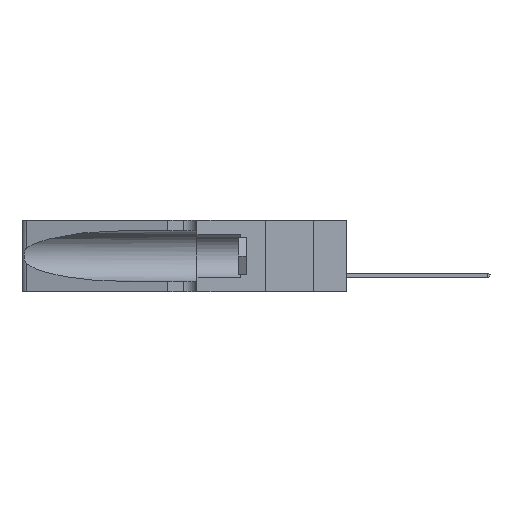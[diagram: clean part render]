
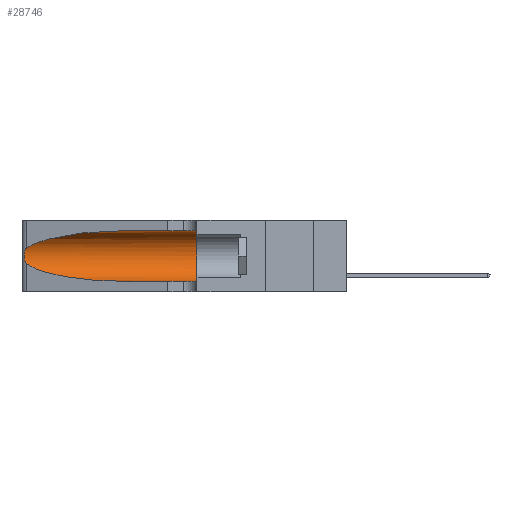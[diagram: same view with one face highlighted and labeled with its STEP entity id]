
A CAD part, left-side view. The second image highlights one B-rep face of the part: STEP entity #28746.
In plain terms, the highlighted cylindrical face has radius 3.308 mm (diameter 6.617 mm), a partial arc.
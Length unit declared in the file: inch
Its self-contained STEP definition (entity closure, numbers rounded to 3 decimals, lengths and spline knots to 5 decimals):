
#509 = DIRECTION ( 'NONE',  ( 0., -1., 0. ) ) ;
#512 = CARTESIAN_POINT ( 'NONE',  ( 0.26017, 1.23833, 0.17102 ) ) ;
#1267 = DIRECTION ( 'NONE',  ( 0., -1., 0. ) ) ;
#1362 = CARTESIAN_POINT ( 'NONE',  ( 0.1305, 1.61858, 0.05475 ) ) ;
#1615 = LINE ( 'NONE', #1362, #5731 ) ;
#3659 = VERTEX_POINT ( 'NONE', #7584 ) ;
#4098 = CARTESIAN_POINT ( 'NONE',  ( 0.1305, 0.35, 0.185 ) ) ;
#4295 = CARTESIAN_POINT ( 'NONE',  ( 0.1305, 0.72297, 0.05475 ) ) ;
#5351 = CARTESIAN_POINT ( 'NONE',  ( 0.25555, 1.22993, 0.14849 ) ) ;
#5681 = CARTESIAN_POINT ( 'NONE',  ( 0.25487, 1.22718, 0.14631 ) ) ;
#5731 = VECTOR ( 'NONE', #1267, 39.37008 ) ;
#5906 = CARTESIAN_POINT ( 'NONE',  ( 0.18966, 0.96281, 0.31525 ) ) ;
#6548 = CARTESIAN_POINT ( 'NONE',  ( 0.25487, 1.22718, 0.22369 ) ) ;
#6645 = CARTESIAN_POINT ( 'NONE',  ( 0.25487, 1.22718, 0.22369 ) ) ;
#6661 =( BOUNDED_CURVE ( )  B_SPLINE_CURVE ( 3, ( #11245, #25977, #30340, #23454 ),
 .UNSPECIFIED., .F., .F. ) 
 B_SPLINE_CURVE_WITH_KNOTS ( ( 4, 4 ),
 ( 3.44316, 4.71239 ),
 .UNSPECIFIED. ) 
 CURVE ( )  GEOMETRIC_REPRESENTATION_ITEM ( )  RATIONAL_B_SPLINE_CURVE ( ( 1., 0.87, 0.87, 1. ) ) 
 REPRESENTATION_ITEM ( '' )  );
#7372 = EDGE_CURVE ( 'NONE', #8222, #18254, #1615, .T. ) ;
#7583 = DIRECTION ( 'NONE',  ( 0., -1., 0. ) ) ;
#7584 = CARTESIAN_POINT ( 'NONE',  ( 0.1305, 0.72297, 0.31525 ) ) ;
#7926 = VERTEX_POINT ( 'NONE', #17925 ) ;
#7997 = B_SPLINE_CURVE_WITH_KNOTS ( 'NONE', 3,
 ( #20129, #29622, #8077, #29407, #24734, #20240, #10627, #27500, #512, #15218, #17430, #19833, #5351, #22248 ),
 .UNSPECIFIED., .F., .F.,
 ( 4, 2, 2, 2, 2, 2, 4 ),
 ( 0., 0.00027, 0.00053, 0.00107, 0.0016, 0.00187, 0.00214 ),
 .UNSPECIFIED. ) ;
#8077 = CARTESIAN_POINT ( 'NONE',  ( 0.25639, 1.23184, 0.21858 ) ) ;
#8222 = VERTEX_POINT ( 'NONE', #4295 ) ;
#9185 = DIRECTION ( 'NONE',  ( 0., 0., 1. ) ) ;
#9838 = CIRCLE ( 'NONE', #19129, 0.13025 ) ;
#10627 = CARTESIAN_POINT ( 'NONE',  ( 0.26075, 1.23896, 0.19203 ) ) ;
#11001 = EDGE_LOOP ( 'NONE', ( #23347, #20241, #25764, #13788, #19202, #22030 ) ) ;
#11118 = CARTESIAN_POINT ( 'NONE',  ( 0.2373, 1.15595, 0.28018 ) ) ;
#11245 = CARTESIAN_POINT ( 'NONE',  ( 0.25487, 1.22718, 0.14631 ) ) ;
#11784 = VECTOR ( 'NONE', #7583, 39.37008 ) ;
#11915 = EDGE_CURVE ( 'NONE', #3659, #26910, #13257, .T. ) ;
#13227 = AXIS2_PLACEMENT_3D ( 'NONE', #21942, #509, #29207 ) ;
#13257 =( BOUNDED_CURVE ( )  B_SPLINE_CURVE ( 3, ( #15792, #5906, #11118, #6548 ),
 .UNSPECIFIED., .F., .F. ) 
 B_SPLINE_CURVE_WITH_KNOTS ( ( 4, 4 ),
 ( 1.5708, 2.84003 ),
 .UNSPECIFIED. ) 
 CURVE ( )  GEOMETRIC_REPRESENTATION_ITEM ( )  RATIONAL_B_SPLINE_CURVE ( ( 1., 0.87, 0.87, 1. ) ) 
 REPRESENTATION_ITEM ( '' )  );
#13788 = ORIENTED_EDGE ( 'NONE', *, *, #7372, .T. ) ;
#14807 = LINE ( 'NONE', #19572, #11784 ) ;
#15218 = CARTESIAN_POINT ( 'NONE',  ( 0.25856, 1.23593, 0.16098 ) ) ;
#15762 = CYLINDRICAL_SURFACE ( 'NONE', #13227, 0.13025 ) ;
#15792 = CARTESIAN_POINT ( 'NONE',  ( 0.1305, 0.72297, 0.31525 ) ) ;
#16594 = EDGE_CURVE ( 'NONE', #3659, #7926, #14807, .T. ) ;
#17063 = VERTEX_POINT ( 'NONE', #5681 ) ;
#17430 = CARTESIAN_POINT ( 'NONE',  ( 0.25789, 1.23486, 0.15765 ) ) ;
#17925 = CARTESIAN_POINT ( 'NONE',  ( 0.1305, 0.35, 0.31525 ) ) ;
#18254 = VERTEX_POINT ( 'NONE', #21851 ) ;
#19129 = AXIS2_PLACEMENT_3D ( 'NONE', #4098, #21222, #9185 ) ;
#19202 = ORIENTED_EDGE ( 'NONE', *, *, #22915, .F. ) ;
#19572 = CARTESIAN_POINT ( 'NONE',  ( 0.1305, 1.61858, 0.31525 ) ) ;
#19833 = CARTESIAN_POINT ( 'NONE',  ( 0.25639, 1.23186, 0.15144 ) ) ;
#20129 = CARTESIAN_POINT ( 'NONE',  ( 0.25487, 1.22718, 0.22369 ) ) ;
#20240 = CARTESIAN_POINT ( 'NONE',  ( 0.26018, 1.23835, 0.19895 ) ) ;
#20241 = ORIENTED_EDGE ( 'NONE', *, *, #30714, .T. ) ;
#21222 = DIRECTION ( 'NONE',  ( 0., 1., 0. ) ) ;
#21851 = CARTESIAN_POINT ( 'NONE',  ( 0.1305, 0.35, 0.05475 ) ) ;
#21942 = CARTESIAN_POINT ( 'NONE',  ( 0.1305, 1.61858, 0.185 ) ) ;
#22030 = ORIENTED_EDGE ( 'NONE', *, *, #16594, .F. ) ;
#22127 = FACE_OUTER_BOUND ( 'NONE', #11001, .T. ) ;
#22248 = CARTESIAN_POINT ( 'NONE',  ( 0.25487, 1.22718, 0.14631 ) ) ;
#22915 = EDGE_CURVE ( 'NONE', #7926, #18254, #9838, .T. ) ;
#23347 = ORIENTED_EDGE ( 'NONE', *, *, #11915, .T. ) ;
#23454 = CARTESIAN_POINT ( 'NONE',  ( 0.1305, 0.72297, 0.05475 ) ) ;
#24027 = EDGE_CURVE ( 'NONE', #17063, #8222, #6661, .T. ) ;
#24734 = CARTESIAN_POINT ( 'NONE',  ( 0.25854, 1.2359, 0.20912 ) ) ;
#25764 = ORIENTED_EDGE ( 'NONE', *, *, #24027, .T. ) ;
#25977 = CARTESIAN_POINT ( 'NONE',  ( 0.2373, 1.15595, 0.08982 ) ) ;
#26910 = VERTEX_POINT ( 'NONE', #6645 ) ;
#27500 = CARTESIAN_POINT ( 'NONE',  ( 0.26075, 1.23896, 0.178 ) ) ;
#28746 = ADVANCED_FACE ( 'NONE', ( #22127 ), #15762, .F. ) ;
#29207 = DIRECTION ( 'NONE',  ( 0., 0., -1. ) ) ;
#29407 = CARTESIAN_POINT ( 'NONE',  ( 0.25787, 1.23484, 0.2124 ) ) ;
#29622 = CARTESIAN_POINT ( 'NONE',  ( 0.25555, 1.22994, 0.2215 ) ) ;
#30340 = CARTESIAN_POINT ( 'NONE',  ( 0.18966, 0.96281, 0.05475 ) ) ;
#30714 = EDGE_CURVE ( 'NONE', #26910, #17063, #7997, .T. ) ;
